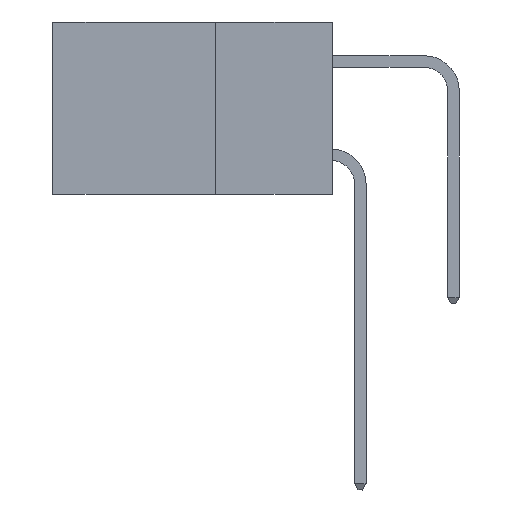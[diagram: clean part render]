
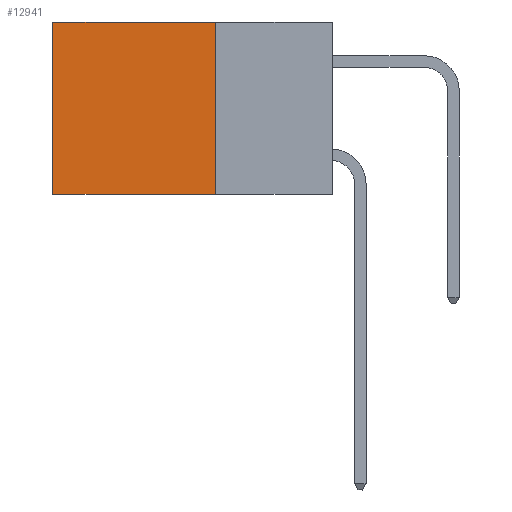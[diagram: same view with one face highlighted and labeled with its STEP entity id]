
A CAD part, left-side view. The second image highlights one B-rep face of the part: STEP entity #12941.
In plain terms, the highlighted planar face has unit normal (-1, 0, 0).
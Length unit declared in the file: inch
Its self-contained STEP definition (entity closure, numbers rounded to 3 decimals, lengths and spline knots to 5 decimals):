
#112 = VERTEX_POINT ( 'NONE', #18784 ) ;
#348 = VECTOR ( 'NONE', #20352, 39.37008 ) ;
#1009 = CARTESIAN_POINT ( 'NONE',  ( 0.2615, 0.25, -0.37 ) ) ;
#1321 = ORIENTED_EDGE ( 'NONE', *, *, #19754, .F. ) ;
#1439 = VECTOR ( 'NONE', #12916, 39.37008 ) ;
#2668 = VERTEX_POINT ( 'NONE', #5726 ) ;
#2844 = VERTEX_POINT ( 'NONE', #15024 ) ;
#3849 = LINE ( 'NONE', #5912, #1439 ) ;
#3875 = CARTESIAN_POINT ( 'NONE',  ( 0.2615, 0.25, 0. ) ) ;
#4273 = ORIENTED_EDGE ( 'NONE', *, *, #19615, .T. ) ;
#4550 = VERTEX_POINT ( 'NONE', #3875 ) ;
#4579 = PLANE ( 'NONE',  #21637 ) ;
#5726 = CARTESIAN_POINT ( 'NONE',  ( 0.2615, 0.6, 0. ) ) ;
#5912 = CARTESIAN_POINT ( 'NONE',  ( 0.2615, 0.25, -0.37 ) ) ;
#6722 = DIRECTION ( 'NONE',  ( 0., 1., 0. ) ) ;
#8351 = VECTOR ( 'NONE', #6722, 39.37008 ) ;
#8757 = LINE ( 'NONE', #11976, #10620 ) ;
#9682 = LINE ( 'NONE', #20121, #348 ) ;
#9728 = DIRECTION ( 'NONE',  ( 0., 0., -1. ) ) ;
#10620 = VECTOR ( 'NONE', #13705, 39.37008 ) ;
#11532 = ORIENTED_EDGE ( 'NONE', *, *, #17473, .T. ) ;
#11976 = CARTESIAN_POINT ( 'NONE',  ( 0.2615, 0.25, -0.37 ) ) ;
#12647 = FACE_OUTER_BOUND ( 'NONE', #19865, .T. ) ;
#12916 = DIRECTION ( 'NONE',  ( 0., 1., 0. ) ) ;
#12941 = ADVANCED_FACE ( 'NONE', ( #12647 ), #4579, .F. ) ;
#13302 = DIRECTION ( 'NONE',  ( 1., 0., 0. ) ) ;
#13705 = DIRECTION ( 'NONE',  ( 0., 0., -1. ) ) ;
#15024 = CARTESIAN_POINT ( 'NONE',  ( 0.2615, 0.25, -0.37 ) ) ;
#17132 = ORIENTED_EDGE ( 'NONE', *, *, #19456, .F. ) ;
#17473 = EDGE_CURVE ( 'NONE', #4550, #2668, #20500, .T. ) ;
#18784 = CARTESIAN_POINT ( 'NONE',  ( 0.2615, 0.6, -0.37 ) ) ;
#19000 = CARTESIAN_POINT ( 'NONE',  ( 0.2615, 0.25, 0. ) ) ;
#19456 = EDGE_CURVE ( 'NONE', #2844, #112, #3849, .T. ) ;
#19615 = EDGE_CURVE ( 'NONE', #2668, #112, #9682, .T. ) ;
#19754 = EDGE_CURVE ( 'NONE', #4550, #2844, #8757, .T. ) ;
#19865 = EDGE_LOOP ( 'NONE', ( #4273, #17132, #1321, #11532 ) ) ;
#20121 = CARTESIAN_POINT ( 'NONE',  ( 0.2615, 0.6, -0.37 ) ) ;
#20352 = DIRECTION ( 'NONE',  ( 0., 0., -1. ) ) ;
#20500 = LINE ( 'NONE', #19000, #8351 ) ;
#21637 = AXIS2_PLACEMENT_3D ( 'NONE', #1009, #13302, #9728 ) ;
